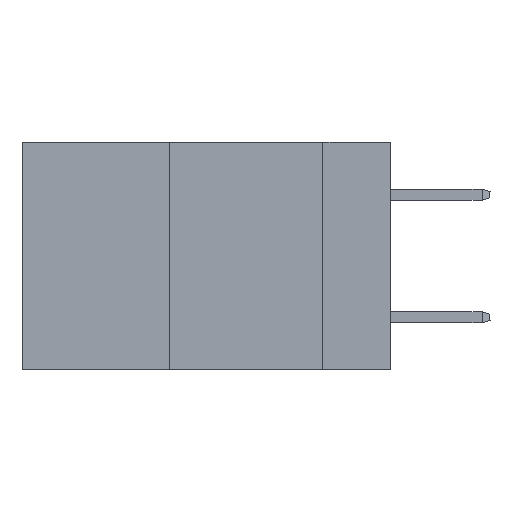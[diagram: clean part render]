
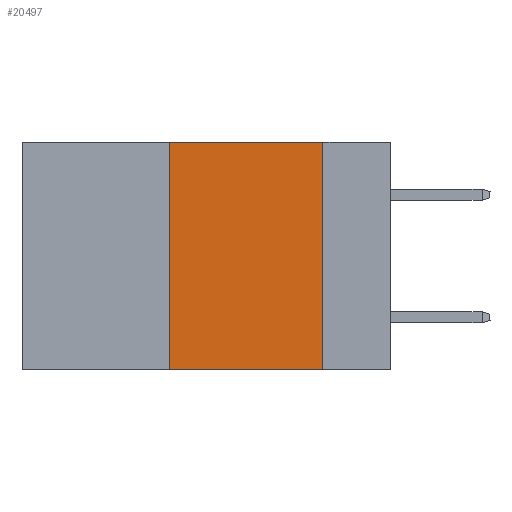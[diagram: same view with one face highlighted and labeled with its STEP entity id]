
A CAD part, left-side view. The second image highlights one B-rep face of the part: STEP entity #20497.
In plain terms, the highlighted planar face has unit normal (-1, 0, 0).
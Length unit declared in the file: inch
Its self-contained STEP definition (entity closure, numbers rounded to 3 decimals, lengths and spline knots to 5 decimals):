
#361 = DIRECTION ( 'NONE',  ( 0., 0., 1. ) ) ;
#2530 = ORIENTED_EDGE ( 'NONE', *, *, #9903, .F. ) ;
#2823 = LINE ( 'NONE', #18982, #18377 ) ;
#3120 = VERTEX_POINT ( 'NONE', #28169 ) ;
#6021 = LINE ( 'NONE', #18239, #27335 ) ;
#6074 = VERTEX_POINT ( 'NONE', #23110 ) ;
#6549 = CARTESIAN_POINT ( 'NONE',  ( 0., 0.6, 0. ) ) ;
#6851 = ORIENTED_EDGE ( 'NONE', *, *, #9535, .F. ) ;
#8740 = CARTESIAN_POINT ( 'NONE',  ( 0., 0.11, -0.37 ) ) ;
#9317 = VECTOR ( 'NONE', #23101, 39.37008 ) ;
#9535 = EDGE_CURVE ( 'NONE', #28077, #6074, #6021, .T. ) ;
#9903 = EDGE_CURVE ( 'NONE', #3120, #24925, #2823, .T. ) ;
#12370 = LINE ( 'NONE', #25940, #15132 ) ;
#12771 = LINE ( 'NONE', #16760, #9317 ) ;
#15132 = VECTOR ( 'NONE', #17395, 39.37008 ) ;
#15167 = AXIS2_PLACEMENT_3D ( 'NONE', #6549, #24329, #19906 ) ;
#16609 = ORIENTED_EDGE ( 'NONE', *, *, #20272, .F. ) ;
#16760 = CARTESIAN_POINT ( 'NONE',  ( 0., 0.6, -0.37 ) ) ;
#16838 = FACE_OUTER_BOUND ( 'NONE', #25325, .T. ) ;
#17100 = ORIENTED_EDGE ( 'NONE', *, *, #18837, .T. ) ;
#17230 = PLANE ( 'NONE',  #15167 ) ;
#17395 = DIRECTION ( 'NONE',  ( 0., -1., 0. ) ) ;
#18239 = CARTESIAN_POINT ( 'NONE',  ( 0., 0.36, 0. ) ) ;
#18377 = VECTOR ( 'NONE', #27998, 39.37008 ) ;
#18837 = EDGE_CURVE ( 'NONE', #28077, #24925, #12771, .T. ) ;
#18982 = CARTESIAN_POINT ( 'NONE',  ( 0., 0.11, 0. ) ) ;
#19906 = DIRECTION ( 'NONE',  ( 0., 0., -1. ) ) ;
#20272 = EDGE_CURVE ( 'NONE', #6074, #3120, #12370, .T. ) ;
#20497 = ADVANCED_FACE ( 'NONE', ( #16838 ), #17230, .F. ) ;
#22311 = CARTESIAN_POINT ( 'NONE',  ( 0., 0.36, -0.37 ) ) ;
#23101 = DIRECTION ( 'NONE',  ( 0., -1., 0. ) ) ;
#23110 = CARTESIAN_POINT ( 'NONE',  ( 0., 0.36, 0. ) ) ;
#24329 = DIRECTION ( 'NONE',  ( 1., 0., 0. ) ) ;
#24925 = VERTEX_POINT ( 'NONE', #8740 ) ;
#25325 = EDGE_LOOP ( 'NONE', ( #2530, #16609, #6851, #17100 ) ) ;
#25940 = CARTESIAN_POINT ( 'NONE',  ( 0., 0.6, 0. ) ) ;
#27335 = VECTOR ( 'NONE', #361, 39.37008 ) ;
#27998 = DIRECTION ( 'NONE',  ( 0., 0., -1. ) ) ;
#28077 = VERTEX_POINT ( 'NONE', #22311 ) ;
#28169 = CARTESIAN_POINT ( 'NONE',  ( 0., 0.11, 0. ) ) ;
